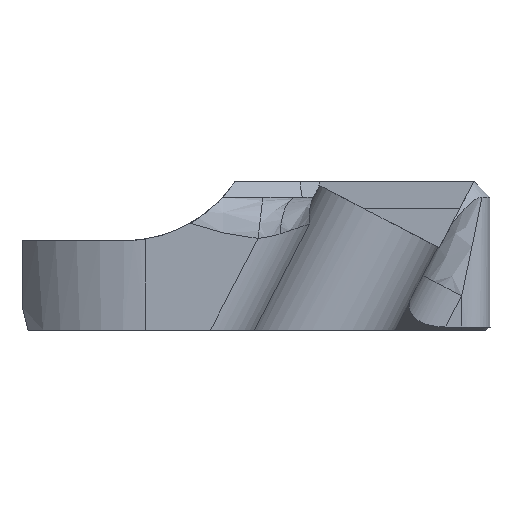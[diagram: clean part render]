
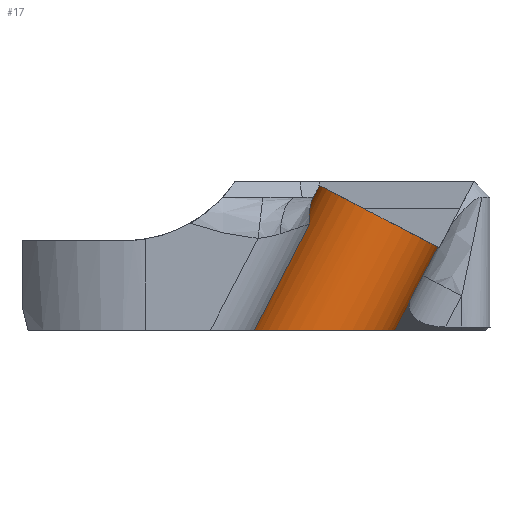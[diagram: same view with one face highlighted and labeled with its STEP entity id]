
A CAD part, front view. The second image highlights one B-rep face of the part: STEP entity #17.
In plain terms, the highlighted cylindrical face has radius 9.525 mm (diameter 19.05 mm), a partial arc.
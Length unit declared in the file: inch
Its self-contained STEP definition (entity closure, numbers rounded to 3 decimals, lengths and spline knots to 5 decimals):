
#17 = ADVANCED_FACE ( 'NONE', ( #8226 ), #5302, .T. ) ;
#54 = VERTEX_POINT ( 'NONE', #1915 ) ;
#172 = CARTESIAN_POINT ( 'NONE',  ( 4.28734, -0.45521, 3.72685 ) ) ;
#318 = ORIENTED_EDGE ( 'NONE', *, *, #1817, .T. ) ;
#455 = CARTESIAN_POINT ( 'NONE',  ( 3.58083, -0.41031, 3.98799 ) ) ;
#498 = CARTESIAN_POINT ( 'NONE',  ( 3.566, -0.53943, 3.91048 ) ) ;
#534 = CARTESIAN_POINT ( 'NONE',  ( 3.56591, -0.59023, 3.85969 ) ) ;
#622 = CARTESIAN_POINT ( 'NONE',  ( 4.04743, -0.41031, 3.25964 ) ) ;
#745 = ORIENTED_EDGE ( 'NONE', *, *, #3512, .F. ) ;
#853 = B_SPLINE_CURVE_WITH_KNOTS ( 'NONE', 3,
 ( #3359, #4888, #2128, #172 ),
 .UNSPECIFIED., .F., .F.,
 ( 4, 4 ),
 ( 0., 0.0046 ),
 .UNSPECIFIED. ) ;
#1009 = VERTEX_POINT ( 'NONE', #6429 ) ;
#1083 = CARTESIAN_POINT ( 'NONE',  ( 3.56566, -0.5805, 3.87033 ) ) ;
#1169 = CARTESIAN_POINT ( 'NONE',  ( 3.5667, -0.52471, 3.92283 ) ) ;
#1817 = EDGE_CURVE ( 'NONE', #8070, #2784, #6192, .T. ) ;
#1818 = DIRECTION ( 'NONE',  ( 0.461, 0., 0.887 ) ) ;
#1879 = ORIENTED_EDGE ( 'NONE', *, *, #3970, .T. ) ;
#1915 = CARTESIAN_POINT ( 'NONE',  ( 4.20316, -0.46052, 3.56645 ) ) ;
#2062 = CARTESIAN_POINT ( 'NONE',  ( 3.43597, -0.59335, 3.606 ) ) ;
#2066 = DIRECTION ( 'NONE',  ( 0.461, 0., 0.887 ) ) ;
#2128 = CARTESIAN_POINT ( 'NONE',  ( 4.25912, -0.45882, 3.67353 ) ) ;
#2159 = VERTEX_POINT ( 'NONE', #455 ) ;
#2639 = CARTESIAN_POINT ( 'NONE',  ( 4.13157, -0.46052, 3.42876 ) ) ;
#2710 = CARTESIAN_POINT ( 'NONE',  ( 4.04743, -0.89273, 3.25964 ) ) ;
#2784 = VERTEX_POINT ( 'NONE', #4826 ) ;
#2813 = DIRECTION ( 'NONE',  ( 0.461, 0., 0.887 ) ) ;
#2825 = LINE ( 'NONE', #3986, #4334 ) ;
#2974 = CARTESIAN_POINT ( 'NONE',  ( 3.57419, -0.44598, 3.97523 ) ) ;
#3088 = DIRECTION ( 'NONE',  ( 0.461, 0., 0.887 ) ) ;
#3277 = CARTESIAN_POINT ( 'NONE',  ( 4.04743, -0.41031, 3.25964 ) ) ;
#3359 = CARTESIAN_POINT ( 'NONE',  ( 4.20316, -0.46052, 3.56645 ) ) ;
#3511 = EDGE_CURVE ( 'NONE', #2159, #7664, #2825, .T. ) ;
#3512 = EDGE_CURVE ( 'NONE', #7664, #1009, #8204, .T. ) ;
#3658 = CARTESIAN_POINT ( 'NONE',  ( 3.56553, -0.56724, 3.88413 ) ) ;
#3724 = CARTESIAN_POINT ( 'NONE',  ( 3.72635, -0.41031, 3.45501 ) ) ;
#3808 = LINE ( 'NONE', #7701, #4058 ) ;
#3889 = EDGE_CURVE ( 'NONE', #6292, #5671, #3808, .T. ) ;
#3930 = EDGE_LOOP ( 'NONE', ( #4796, #7920, #745, #6415, #6123, #318, #5482, #6130, #1879 ) ) ;
#3970 = EDGE_CURVE ( 'NONE', #5671, #4093, #4013, .T. ) ;
#3986 = CARTESIAN_POINT ( 'NONE',  ( 3.39364, -0.41031, 3.62801 ) ) ;
#4013 =( BOUNDED_CURVE ( )  B_SPLINE_CURVE ( 3, ( #5875, #5813, #5779, #2639 ),
 .UNSPECIFIED., .F., .F. ) 
 B_SPLINE_CURVE_WITH_KNOTS ( ( 4, 4 ),
 ( 5.29498, 5.42926 ),
 .UNSPECIFIED. ) 
 CURVE ( )  GEOMETRIC_REPRESENTATION_ITEM ( )  RATIONAL_B_SPLINE_CURVE ( ( 1., 0.998, 0.998, 1. ) ) 
 REPRESENTATION_ITEM ( '' )  );
#4058 = VECTOR ( 'NONE', #3088, 39.37008 ) ;
#4093 = VERTEX_POINT ( 'NONE', #6538 ) ;
#4240 = EDGE_CURVE ( 'NONE', #6292, #2784, #4908, .T. ) ;
#4306 = CARTESIAN_POINT ( 'NONE',  ( 3.56604, -0.59335, 3.85614 ) ) ;
#4334 = VECTOR ( 'NONE', #4624, 39.37008 ) ;
#4336 = EDGE_CURVE ( 'NONE', #54, #1009, #853, .T. ) ;
#4361 = EDGE_CURVE ( 'NONE', #4093, #54, #5304, .T. ) ;
#4519 = CARTESIAN_POINT ( 'NONE',  ( 3.62432, -0.41031, 4.07162 ) ) ;
#4526 = CARTESIAN_POINT ( 'NONE',  ( 4.11709, -0.41031, 3.39361 ) ) ;
#4565 = EDGE_CURVE ( 'NONE', #2159, #8070, #7968, .T. ) ;
#4624 = DIRECTION ( 'NONE',  ( 0.461, 0., 0.887 ) ) ;
#4711 = CARTESIAN_POINT ( 'NONE',  ( 3.56604, -0.59335, 3.85614 ) ) ;
#4796 = ORIENTED_EDGE ( 'NONE', *, *, #4361, .T. ) ;
#4826 = CARTESIAN_POINT ( 'NONE',  ( 3.25586, -0.59335, 3.25964 ) ) ;
#4888 = CARTESIAN_POINT ( 'NONE',  ( 4.23104, -0.46052, 3.62007 ) ) ;
#4908 =( BOUNDED_CURVE ( )  B_SPLINE_CURVE ( 3, ( #3277, #2710, #6559, #5295 ),
 .UNSPECIFIED., .F., .F. ) 
 B_SPLINE_CURVE_WITH_KNOTS ( ( 4, 4 ),
 ( 0., 2.63168 ),
 .UNSPECIFIED. ) 
 CURVE ( )  GEOMETRIC_REPRESENTATION_ITEM ( )  RATIONAL_B_SPLINE_CURVE ( ( 1., 0.501, 0.501, 1. ) ) 
 REPRESENTATION_ITEM ( '' )  );
#5295 = CARTESIAN_POINT ( 'NONE',  ( 3.25586, -0.59335, 3.25964 ) ) ;
#5302 = CYLINDRICAL_SURFACE ( 'NONE', #8003, 0.375 ) ;
#5304 = LINE ( 'NONE', #6641, #8039 ) ;
#5482 = ORIENTED_EDGE ( 'NONE', *, *, #4240, .F. ) ;
#5671 = VERTEX_POINT ( 'NONE', #4526 ) ;
#5779 = CARTESIAN_POINT ( 'NONE',  ( 4.12804, -0.44387, 3.41711 ) ) ;
#5813 = CARTESIAN_POINT ( 'NONE',  ( 4.12321, -0.42711, 3.40537 ) ) ;
#5875 = CARTESIAN_POINT ( 'NONE',  ( 4.11709, -0.41031, 3.39361 ) ) ;
#5915 = DIRECTION ( 'NONE',  ( 0.887, 0., -0.461 ) ) ;
#6123 = ORIENTED_EDGE ( 'NONE', *, *, #4565, .T. ) ;
#6130 = ORIENTED_EDGE ( 'NONE', *, *, #3889, .T. ) ;
#6192 = LINE ( 'NONE', #2062, #6999 ) ;
#6277 = CARTESIAN_POINT ( 'NONE',  ( 3.56557, -0.56042, 3.89086 ) ) ;
#6290 = DIRECTION ( 'NONE',  ( 0.887, 0., -0.461 ) ) ;
#6292 = VERTEX_POINT ( 'NONE', #622 ) ;
#6415 = ORIENTED_EDGE ( 'NONE', *, *, #3511, .F. ) ;
#6429 = CARTESIAN_POINT ( 'NONE',  ( 4.28734, -0.45521, 3.72685 ) ) ;
#6433 = AXIS2_PLACEMENT_3D ( 'NONE', #7192, #2066, #5915 ) ;
#6538 = CARTESIAN_POINT ( 'NONE',  ( 4.13157, -0.46052, 3.42876 ) ) ;
#6559 = CARTESIAN_POINT ( 'NONE',  ( 3.52126, -1.0144, 3.25964 ) ) ;
#6641 = CARTESIAN_POINT ( 'NONE',  ( 4.05606, -0.46052, 3.28356 ) ) ;
#6999 = VECTOR ( 'NONE', #8126, 39.37008 ) ;
#7192 = CARTESIAN_POINT ( 'NONE',  ( 3.95702, -0.41031, 3.89861 ) ) ;
#7554 = CARTESIAN_POINT ( 'NONE',  ( 3.58083, -0.41031, 3.98799 ) ) ;
#7584 = CARTESIAN_POINT ( 'NONE',  ( 3.56561, -0.57722, 3.87381 ) ) ;
#7664 = VERTEX_POINT ( 'NONE', #4519 ) ;
#7701 = CARTESIAN_POINT ( 'NONE',  ( 4.05905, -0.41031, 3.282 ) ) ;
#7920 = ORIENTED_EDGE ( 'NONE', *, *, #4336, .T. ) ;
#7968 = B_SPLINE_CURVE_WITH_KNOTS ( 'NONE', 3,
 ( #7554, #2974, #8175, #1169, #498, #6277, #3658, #7584, #1083, #8201, #534, #4306 ),
 .UNSPECIFIED., .F., .F.,
 ( 4, 2, 2, 2, 2, 4 ),
 ( 0., 0.00288, 0.00432, 0.00504, 0.00541, 0.00577 ),
 .UNSPECIFIED. ) ;
#8003 = AXIS2_PLACEMENT_3D ( 'NONE', #3724, #1818, #6290 ) ;
#8039 = VECTOR ( 'NONE', #2813, 39.37008 ) ;
#8070 = VERTEX_POINT ( 'NONE', #4711 ) ;
#8126 = DIRECTION ( 'NONE',  ( -0.461, 0., -0.887 ) ) ;
#8175 = CARTESIAN_POINT ( 'NONE',  ( 3.57015, -0.47876, 3.95677 ) ) ;
#8201 = CARTESIAN_POINT ( 'NONE',  ( 3.56581, -0.58699, 3.86329 ) ) ;
#8204 = CIRCLE ( 'NONE', #6433, 0.375 ) ;
#8226 = FACE_OUTER_BOUND ( 'NONE', #3930, .T. ) ;
